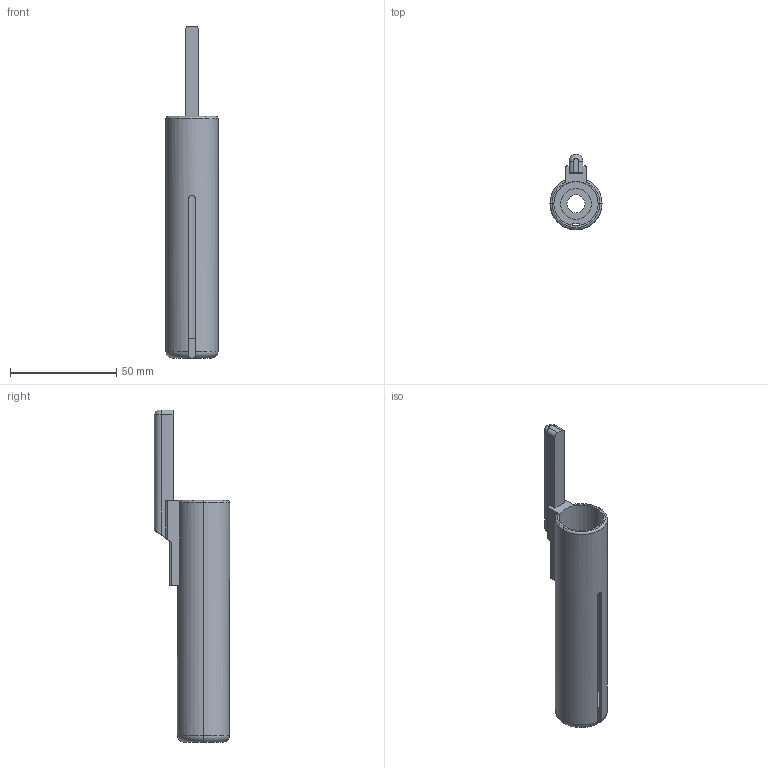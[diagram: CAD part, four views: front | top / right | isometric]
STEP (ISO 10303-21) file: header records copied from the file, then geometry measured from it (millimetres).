
FILE_DESCRIPTION (( 'STEP AP203' ), '1' );
FILE_NAME ('boltcarrier.STEP', '2021-12-29T04:12:51', ( '' ), ( '' ), 'SwSTEP 2.0', 'SolidWorks 2015', '' );
FILE_SCHEMA (( 'CONFIG_CONTROL_DESIGN' ));
Length unit declared in the file: millimetre
Products named in the file (1): boltcarrier
Bounding box: 24.5 x 35.31 x 156 mm (x, y, z)
Volume: 20963.8 mm3; surface area: 18338.6 mm2
Topology: 1 solids, 1 shells, 41 faces, 110 edges, 71 vertices
Faces by surface type: plane 18, cylinder 16, torus 7
Entity records: 1471 total; most frequent: CARTESIAN_POINT 352, DIRECTION 221, ORIENTED_EDGE 220, EDGE_CURVE 110, AXIS2_PLACEMENT_3D 82, VERTEX_POINT 71, LINE 57, VECTOR 57
